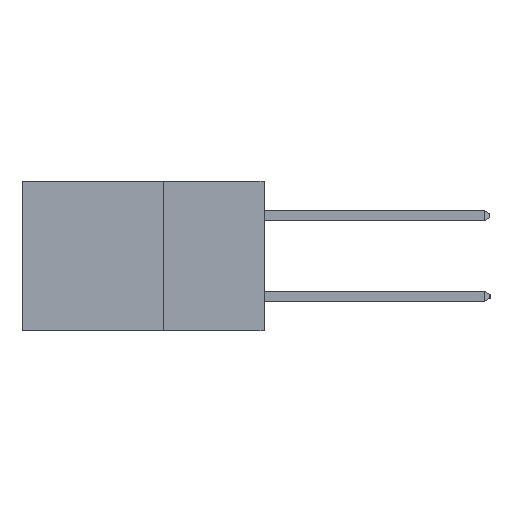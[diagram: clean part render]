
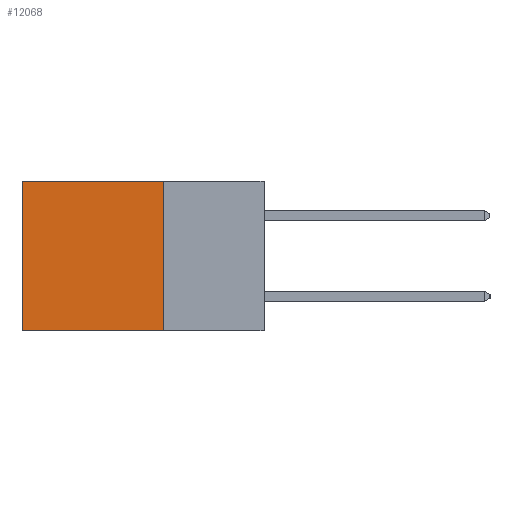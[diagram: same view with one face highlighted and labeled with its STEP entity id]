
A CAD part, left-side view. The second image highlights one B-rep face of the part: STEP entity #12068.
In plain terms, the highlighted planar face has unit normal (-1, 0, 0).
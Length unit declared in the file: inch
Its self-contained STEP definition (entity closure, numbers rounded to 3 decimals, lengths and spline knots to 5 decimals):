
#51 = CARTESIAN_POINT ( 'NONE',  ( 0.2615, 0.25, 0. ) ) ;
#1060 = EDGE_CURVE ( 'NONE', #2024, #13158, #9513, .T. ) ;
#1788 = EDGE_LOOP ( 'NONE', ( #7320, #9619, #11308, #12553 ) ) ;
#1810 = VECTOR ( 'NONE', #7367, 39.37008 ) ;
#2024 = VERTEX_POINT ( 'NONE', #51 ) ;
#2070 = DIRECTION ( 'NONE',  ( 0., 1., 0. ) ) ;
#2272 = CARTESIAN_POINT ( 'NONE',  ( 0.2615, 0.25, -0.37 ) ) ;
#2451 = AXIS2_PLACEMENT_3D ( 'NONE', #3468, #3529, #12396 ) ;
#2453 = EDGE_CURVE ( 'NONE', #4917, #3910, #14440, .T. ) ;
#3468 = CARTESIAN_POINT ( 'NONE',  ( 0.2615, 0.25, -0.37 ) ) ;
#3494 = EDGE_CURVE ( 'NONE', #2024, #4917, #15626, .T. ) ;
#3529 = DIRECTION ( 'NONE',  ( 1., 0., 0. ) ) ;
#3541 = DIRECTION ( 'NONE',  ( 0., 0., -1. ) ) ;
#3664 = CARTESIAN_POINT ( 'NONE',  ( 0.2615, 0.25, -0.37 ) ) ;
#3901 = VECTOR ( 'NONE', #2070, 39.37008 ) ;
#3910 = VERTEX_POINT ( 'NONE', #6846 ) ;
#4917 = VERTEX_POINT ( 'NONE', #3664 ) ;
#5493 = VECTOR ( 'NONE', #3541, 39.37008 ) ;
#5573 = LINE ( 'NONE', #8595, #1810 ) ;
#6846 = CARTESIAN_POINT ( 'NONE',  ( 0.2615, 0.6, -0.37 ) ) ;
#7320 = ORIENTED_EDGE ( 'NONE', *, *, #13880, .T. ) ;
#7367 = DIRECTION ( 'NONE',  ( 0., 0., -1. ) ) ;
#8438 = CARTESIAN_POINT ( 'NONE',  ( 0.2615, 0.25, -0.37 ) ) ;
#8569 = DIRECTION ( 'NONE',  ( 0., 1., 0. ) ) ;
#8595 = CARTESIAN_POINT ( 'NONE',  ( 0.2615, 0.6, -0.37 ) ) ;
#9513 = LINE ( 'NONE', #16183, #13297 ) ;
#9619 = ORIENTED_EDGE ( 'NONE', *, *, #2453, .F. ) ;
#11099 = PLANE ( 'NONE',  #2451 ) ;
#11308 = ORIENTED_EDGE ( 'NONE', *, *, #3494, .F. ) ;
#12068 = ADVANCED_FACE ( 'NONE', ( #14164 ), #11099, .F. ) ;
#12396 = DIRECTION ( 'NONE',  ( 0., 0., -1. ) ) ;
#12553 = ORIENTED_EDGE ( 'NONE', *, *, #1060, .T. ) ;
#13158 = VERTEX_POINT ( 'NONE', #16178 ) ;
#13297 = VECTOR ( 'NONE', #8569, 39.37008 ) ;
#13880 = EDGE_CURVE ( 'NONE', #13158, #3910, #5573, .T. ) ;
#14164 = FACE_OUTER_BOUND ( 'NONE', #1788, .T. ) ;
#14440 = LINE ( 'NONE', #8438, #3901 ) ;
#15626 = LINE ( 'NONE', #2272, #5493 ) ;
#16178 = CARTESIAN_POINT ( 'NONE',  ( 0.2615, 0.6, 0. ) ) ;
#16183 = CARTESIAN_POINT ( 'NONE',  ( 0.2615, 0.25, 0. ) ) ;
